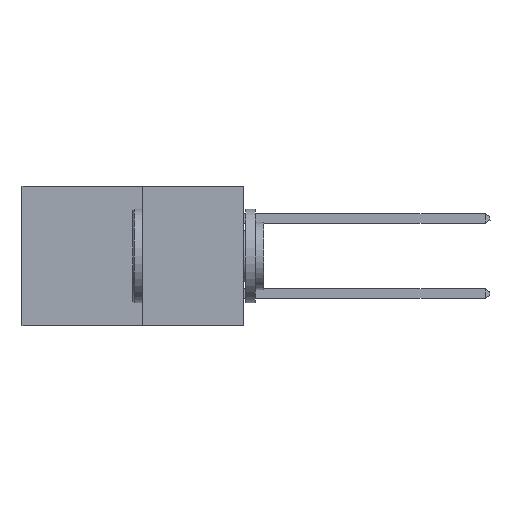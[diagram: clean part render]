
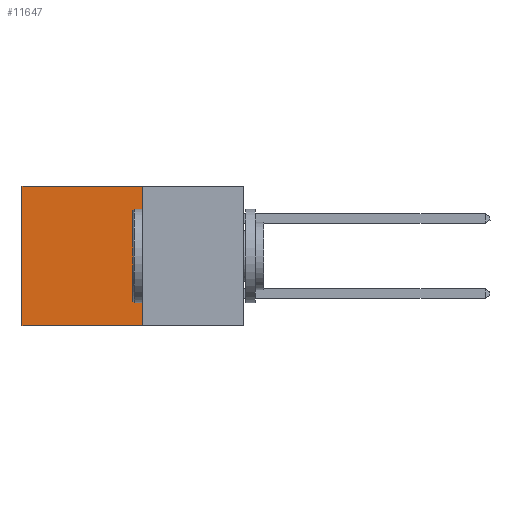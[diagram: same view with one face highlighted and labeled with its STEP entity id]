
A CAD part, left-side view. The second image highlights one B-rep face of the part: STEP entity #11647.
In plain terms, the highlighted planar face has unit normal (-1, 0, 0).
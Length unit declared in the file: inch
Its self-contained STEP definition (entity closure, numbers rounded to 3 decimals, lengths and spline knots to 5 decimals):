
#374 = CARTESIAN_POINT ( 'NONE',  ( 0.277, 0.27, 0. ) ) ;
#571 = EDGE_CURVE ( 'NONE', #7709, #6692, #5427, .T. ) ;
#1129 = CARTESIAN_POINT ( 'NONE',  ( 0.277, 0.27, -0.37 ) ) ;
#1167 = LINE ( 'NONE', #10384, #10729 ) ;
#1192 = CARTESIAN_POINT ( 'NONE',  ( 0.277, 0.27, -0.37 ) ) ;
#1457 = EDGE_CURVE ( 'NONE', #7709, #7623, #11805, .T. ) ;
#1472 = ORIENTED_EDGE ( 'NONE', *, *, #1457, .F. ) ;
#1511 = ORIENTED_EDGE ( 'NONE', *, *, #571, .T. ) ;
#1935 = DIRECTION ( 'NONE',  ( 0., 1., 0. ) ) ;
#1970 = EDGE_LOOP ( 'NONE', ( #3697, #3677, #1472, #1511 ) ) ;
#2109 = VECTOR ( 'NONE', #4973, 39.37008 ) ;
#2174 = PLANE ( 'NONE',  #2301 ) ;
#2301 = AXIS2_PLACEMENT_3D ( 'NONE', #1129, #6787, #8599 ) ;
#2535 = EDGE_CURVE ( 'NONE', #6692, #10299, #1167, .T. ) ;
#3015 = VECTOR ( 'NONE', #3219, 39.37008 ) ;
#3219 = DIRECTION ( 'NONE',  ( 0., 1., 0. ) ) ;
#3677 = ORIENTED_EDGE ( 'NONE', *, *, #9243, .F. ) ;
#3697 = ORIENTED_EDGE ( 'NONE', *, *, #2535, .T. ) ;
#3831 = CARTESIAN_POINT ( 'NONE',  ( 0.277, 0.27, -0.37 ) ) ;
#4973 = DIRECTION ( 'NONE',  ( 0., 0., -1. ) ) ;
#5127 = CARTESIAN_POINT ( 'NONE',  ( 0.277, 0.59, 0. ) ) ;
#5427 = LINE ( 'NONE', #7265, #3015 ) ;
#5776 = FACE_OUTER_BOUND ( 'NONE', #1970, .T. ) ;
#6692 = VERTEX_POINT ( 'NONE', #5127 ) ;
#6787 = DIRECTION ( 'NONE',  ( 1., 0., 0. ) ) ;
#7265 = CARTESIAN_POINT ( 'NONE',  ( 0.277, 0.27, 0. ) ) ;
#7501 = CARTESIAN_POINT ( 'NONE',  ( 0.277, 0.27, -0.37 ) ) ;
#7623 = VERTEX_POINT ( 'NONE', #1192 ) ;
#7709 = VERTEX_POINT ( 'NONE', #374 ) ;
#8599 = DIRECTION ( 'NONE',  ( 0., 0., -1. ) ) ;
#9243 = EDGE_CURVE ( 'NONE', #7623, #10299, #9971, .T. ) ;
#9691 = VECTOR ( 'NONE', #1935, 39.37008 ) ;
#9971 = LINE ( 'NONE', #7501, #9691 ) ;
#10102 = DIRECTION ( 'NONE',  ( 0., 0., -1. ) ) ;
#10299 = VERTEX_POINT ( 'NONE', #10327 ) ;
#10327 = CARTESIAN_POINT ( 'NONE',  ( 0.277, 0.59, -0.37 ) ) ;
#10384 = CARTESIAN_POINT ( 'NONE',  ( 0.277, 0.59, -0.37 ) ) ;
#10729 = VECTOR ( 'NONE', #10102, 39.37008 ) ;
#11647 = ADVANCED_FACE ( 'NONE', ( #5776 ), #2174, .F. ) ;
#11805 = LINE ( 'NONE', #3831, #2109 ) ;
